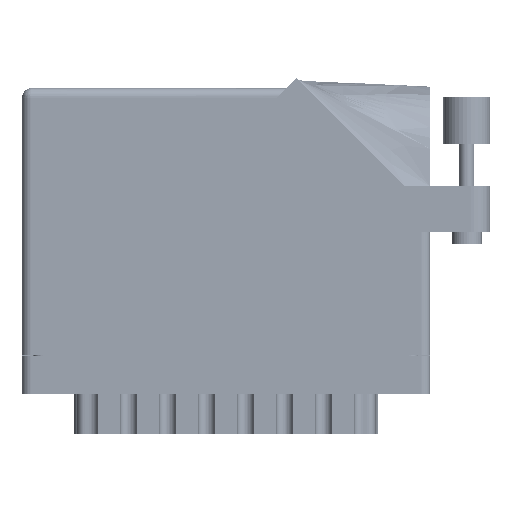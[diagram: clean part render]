
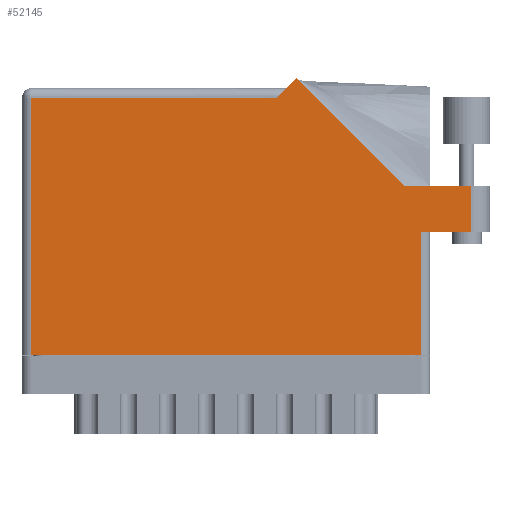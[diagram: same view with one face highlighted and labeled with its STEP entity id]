
A CAD part, front view. The second image highlights one B-rep face of the part: STEP entity #52145.
In plain terms, the highlighted face is planar.
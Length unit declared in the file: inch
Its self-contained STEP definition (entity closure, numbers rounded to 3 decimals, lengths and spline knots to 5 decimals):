
#305 = EDGE_CURVE ( 'NONE', #51995, #24570, #62474, .T. ) ;
#1394 = CARTESIAN_POINT ( 'NONE',  ( 0.062, 1.713, 0. ) ) ;
#2718 = ORIENTED_EDGE ( 'NONE', *, *, #21797, .T. ) ;
#3037 = AXIS2_PLACEMENT_3D ( 'NONE', #51546, #28858, #33800 ) ;
#3114 = EDGE_CURVE ( 'NONE', #48747, #12184, #55216, .T. ) ;
#3586 = CARTESIAN_POINT ( 'NONE',  ( 1.696, 1.713, 0. ) ) ;
#6544 = PLANE ( 'NONE',  #3037 ) ;
#6950 = ORIENTED_EDGE ( 'NONE', *, *, #23119, .T. ) ;
#8474 = CARTESIAN_POINT ( 'NONE',  ( 2.55242, 1.122, 0. ) ) ;
#9500 = ORIENTED_EDGE ( 'NONE', *, *, #30849, .T. ) ;
#11543 = DIRECTION ( 'NONE',  ( -1., 0., 0. ) ) ;
#12184 = VERTEX_POINT ( 'NONE', #1394 ) ;
#12247 = DIRECTION ( 'NONE',  ( -1., 0., 0. ) ) ;
#12542 = VERTEX_POINT ( 'NONE', #27107 ) ;
#13551 = DIRECTION ( 'NONE',  ( -0.707, -0.707, 0. ) ) ;
#15334 = EDGE_LOOP ( 'NONE', ( #54634, #40873, #44420, #2718, #37228, #33268, #68211, #6950, #9500 ) ) ;
#15918 = CARTESIAN_POINT ( 'NONE',  ( 2.993, 1.122, 0. ) ) ;
#15975 = VECTOR ( 'NONE', #18636, 39.37008 ) ;
#17751 = DIRECTION ( 'NONE',  ( 1., 0., 0. ) ) ;
#18636 = DIRECTION ( 'NONE',  ( 0., 1., 0. ) ) ;
#18990 = DIRECTION ( 'NONE',  ( 0., -1., 0. ) ) ;
#19250 = CARTESIAN_POINT ( 'NONE',  ( 0.062, 0., 0. ) ) ;
#21797 = EDGE_CURVE ( 'NONE', #24570, #32773, #60043, .T. ) ;
#22932 = CARTESIAN_POINT ( 'NONE',  ( 2.55242, 1.122, 0. ) ) ;
#23119 = EDGE_CURVE ( 'NONE', #27881, #12542, #59152, .T. ) ;
#23936 = VECTOR ( 'NONE', #46125, 39.37008 ) ;
#24003 = CARTESIAN_POINT ( 'NONE',  ( 2.656, 0.815, 0. ) ) ;
#24393 = DIRECTION ( 'NONE',  ( -0.707, 0.707, 0. ) ) ;
#24570 = VERTEX_POINT ( 'NONE', #8474 ) ;
#25441 = LINE ( 'NONE', #29969, #60677 ) ;
#27107 = CARTESIAN_POINT ( 'NONE',  ( 2.656, 0., 0. ) ) ;
#27881 = VERTEX_POINT ( 'NONE', #69946 ) ;
#28300 = CARTESIAN_POINT ( 'NONE',  ( 1.82871, 1.84571, 0. ) ) ;
#28858 = DIRECTION ( 'NONE',  ( 0., 0., -1. ) ) ;
#29117 = VERTEX_POINT ( 'NONE', #35999 ) ;
#29158 = CARTESIAN_POINT ( 'NONE',  ( 0., 1.713, 0. ) ) ;
#29661 = CARTESIAN_POINT ( 'NONE',  ( 0., 0., 0. ) ) ;
#29969 = CARTESIAN_POINT ( 'NONE',  ( 2.718, 0.815, 0. ) ) ;
#30849 = EDGE_CURVE ( 'NONE', #12542, #35168, #67937, .T. ) ;
#32773 = VERTEX_POINT ( 'NONE', #28300 ) ;
#33268 = ORIENTED_EDGE ( 'NONE', *, *, #3114, .T. ) ;
#33800 = DIRECTION ( 'NONE',  ( -1., 0., 0. ) ) ;
#33919 = VECTOR ( 'NONE', #18990, 39.37008 ) ;
#35168 = VERTEX_POINT ( 'NONE', #46517 ) ;
#35327 = LINE ( 'NONE', #59727, #44957 ) ;
#35999 = CARTESIAN_POINT ( 'NONE',  ( 2.993, 0.815, 0. ) ) ;
#37228 = ORIENTED_EDGE ( 'NONE', *, *, #38971, .T. ) ;
#38971 = EDGE_CURVE ( 'NONE', #32773, #48747, #54869, .T. ) ;
#40202 = VECTOR ( 'NONE', #12247, 39.37008 ) ;
#40873 = ORIENTED_EDGE ( 'NONE', *, *, #53596, .T. ) ;
#41283 = EDGE_CURVE ( 'NONE', #35168, #29117, #25441, .T. ) ;
#41349 = VECTOR ( 'NONE', #11543, 39.37008 ) ;
#44420 = ORIENTED_EDGE ( 'NONE', *, *, #305, .T. ) ;
#44957 = VECTOR ( 'NONE', #71074, 39.37008 ) ;
#46125 = DIRECTION ( 'NONE',  ( 1., 0., 0. ) ) ;
#46517 = CARTESIAN_POINT ( 'NONE',  ( 2.656, 0.815, 0. ) ) ;
#46771 = VECTOR ( 'NONE', #24393, 39.37008 ) ;
#48070 = LINE ( 'NONE', #19250, #33919 ) ;
#48747 = VERTEX_POINT ( 'NONE', #3586 ) ;
#51546 = CARTESIAN_POINT ( 'NONE',  ( 0., 1.775, 0. ) ) ;
#51995 = VERTEX_POINT ( 'NONE', #15918 ) ;
#52145 = ADVANCED_FACE ( 'NONE', ( #70858 ), #6544, .F. ) ;
#53596 = EDGE_CURVE ( 'NONE', #29117, #51995, #35327, .T. ) ;
#54634 = ORIENTED_EDGE ( 'NONE', *, *, #41283, .T. ) ;
#54869 = LINE ( 'NONE', #59057, #67242 ) ;
#55216 = LINE ( 'NONE', #29158, #40202 ) ;
#55515 = EDGE_CURVE ( 'NONE', #12184, #27881, #48070, .T. ) ;
#56758 = CARTESIAN_POINT ( 'NONE',  ( 3.118, 1.122, 0. ) ) ;
#59057 = CARTESIAN_POINT ( 'NONE',  ( 1.758, 1.775, 0. ) ) ;
#59152 = LINE ( 'NONE', #29661, #23936 ) ;
#59727 = CARTESIAN_POINT ( 'NONE',  ( 2.993, 1.122, 0. ) ) ;
#60043 = LINE ( 'NONE', #22932, #46771 ) ;
#60677 = VECTOR ( 'NONE', #17751, 39.37008 ) ;
#62474 = LINE ( 'NONE', #56758, #41349 ) ;
#67242 = VECTOR ( 'NONE', #13551, 39.37008 ) ;
#67937 = LINE ( 'NONE', #24003, #15975 ) ;
#68211 = ORIENTED_EDGE ( 'NONE', *, *, #55515, .T. ) ;
#69946 = CARTESIAN_POINT ( 'NONE',  ( 0.062, 0., 0. ) ) ;
#70858 = FACE_OUTER_BOUND ( 'NONE', #15334, .T. ) ;
#71074 = DIRECTION ( 'NONE',  ( 0., 1., 0. ) ) ;
